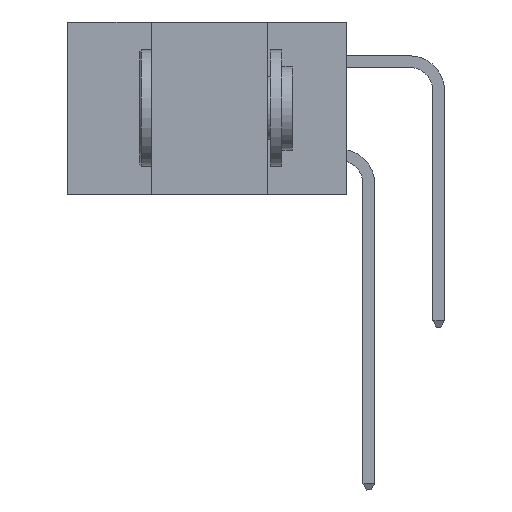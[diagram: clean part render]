
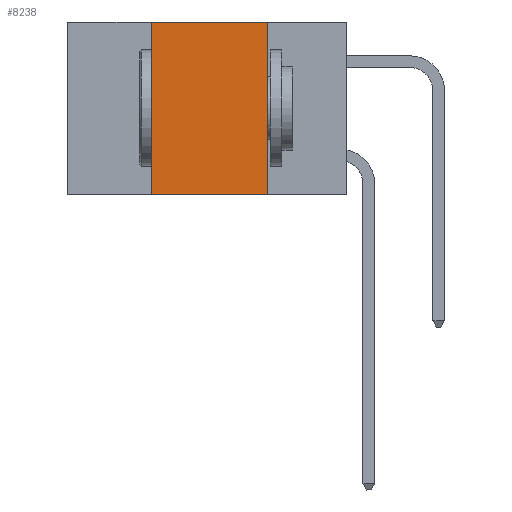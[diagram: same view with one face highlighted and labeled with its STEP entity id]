
A CAD part, left-side view. The second image highlights one B-rep face of the part: STEP entity #8238.
In plain terms, the highlighted planar face has unit normal (-1, 0, 0).
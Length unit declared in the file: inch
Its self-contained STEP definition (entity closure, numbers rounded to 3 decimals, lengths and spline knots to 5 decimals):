
#8 = ORIENTED_EDGE ( 'NONE', *, *, #11877, .T. ) ;
#1325 = PLANE ( 'NONE',  #16401 ) ;
#2678 = ORIENTED_EDGE ( 'NONE', *, *, #5757, .F. ) ;
#3081 = CARTESIAN_POINT ( 'NONE',  ( 0., 0.42, -0.37 ) ) ;
#3141 = VERTEX_POINT ( 'NONE', #5247 ) ;
#3259 = CARTESIAN_POINT ( 'NONE',  ( 0., 0.17, 0. ) ) ;
#4129 = VERTEX_POINT ( 'NONE', #25004 ) ;
#4217 = LINE ( 'NONE', #23497, #14390 ) ;
#5218 = DIRECTION ( 'NONE',  ( 0., 0., 1. ) ) ;
#5247 = CARTESIAN_POINT ( 'NONE',  ( 0., 0.42, 0. ) ) ;
#5705 = DIRECTION ( 'NONE',  ( 0., -1., 0. ) ) ;
#5757 = EDGE_CURVE ( 'NONE', #3141, #17059, #4217, .T. ) ;
#6549 = FACE_OUTER_BOUND ( 'NONE', #12808, .T. ) ;
#6824 = VECTOR ( 'NONE', #5218, 39.37008 ) ;
#7053 = EDGE_CURVE ( 'NONE', #17059, #4129, #7905, .T. ) ;
#7596 = VERTEX_POINT ( 'NONE', #3081 ) ;
#7905 = LINE ( 'NONE', #17685, #24785 ) ;
#8238 = ADVANCED_FACE ( 'NONE', ( #6549 ), #1325, .F. ) ;
#10697 = ORIENTED_EDGE ( 'NONE', *, *, #20580, .F. ) ;
#11532 = DIRECTION ( 'NONE',  ( 0., 0., -1. ) ) ;
#11877 = EDGE_CURVE ( 'NONE', #7596, #4129, #13571, .T. ) ;
#12089 = ORIENTED_EDGE ( 'NONE', *, *, #7053, .F. ) ;
#12808 = EDGE_LOOP ( 'NONE', ( #12089, #2678, #10697, #8 ) ) ;
#13571 = LINE ( 'NONE', #13906, #18002 ) ;
#13906 = CARTESIAN_POINT ( 'NONE',  ( 0., 0.6, -0.37 ) ) ;
#14390 = VECTOR ( 'NONE', #25736, 39.37008 ) ;
#15322 = DIRECTION ( 'NONE',  ( 0., 0., -1. ) ) ;
#15505 = CARTESIAN_POINT ( 'NONE',  ( 0., 0.6, 0. ) ) ;
#15774 = LINE ( 'NONE', #17231, #6824 ) ;
#16401 = AXIS2_PLACEMENT_3D ( 'NONE', #15505, #19587, #15322 ) ;
#17059 = VERTEX_POINT ( 'NONE', #3259 ) ;
#17231 = CARTESIAN_POINT ( 'NONE',  ( 0., 0.42, 0. ) ) ;
#17685 = CARTESIAN_POINT ( 'NONE',  ( 0., 0.17, 0. ) ) ;
#18002 = VECTOR ( 'NONE', #5705, 39.37008 ) ;
#19587 = DIRECTION ( 'NONE',  ( 1., 0., 0. ) ) ;
#20580 = EDGE_CURVE ( 'NONE', #7596, #3141, #15774, .T. ) ;
#23497 = CARTESIAN_POINT ( 'NONE',  ( 0., 0.6, 0. ) ) ;
#24785 = VECTOR ( 'NONE', #11532, 39.37008 ) ;
#25004 = CARTESIAN_POINT ( 'NONE',  ( 0., 0.17, -0.37 ) ) ;
#25736 = DIRECTION ( 'NONE',  ( 0., -1., 0. ) ) ;
